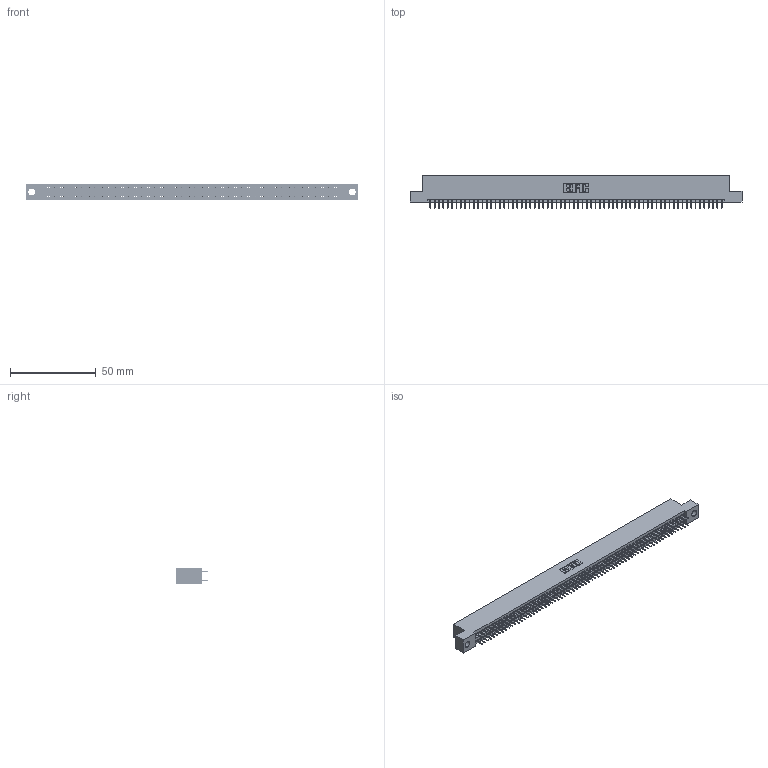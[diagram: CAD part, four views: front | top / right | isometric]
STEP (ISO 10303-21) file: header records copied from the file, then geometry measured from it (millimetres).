
FILE_DESCRIPTION (( 'STEP AP203' ), '1' );
FILE_NAME ('395-136-525-204.STEP', '2020-09-26T03:54:42', ( '' ), ( '' ), 'SwSTEP 2.0', 'SolidWorks 2020', '' );
FILE_SCHEMA (( 'CONFIG_CONTROL_DESIGN' ));
Length unit declared in the file: inch
Products named in the file (3): 345-292-001_345-293-125; 395-136-525-204; 345 Part_Flush Mounting Lugs - 0.156 Dia-TH
Assembly tree (137 placements, depth 2):
  395-136-525-204
    345 Part_Flush Mounting Lugs - 0.156 Dia-TH
    345-292-001_345-293-125  x136
Bounding box: 193.93 x 18.72 x 9.4 mm (x, y, z)
Volume: 18768.1 mm3; surface area: 27386.6 mm2
Topology: 137 solids, 137 shells, 7470 faces, 21149 edges, 13554 vertices
Faces by surface type: plane 5384, cylinder 2086
Entity records: 49931 total; most frequent: CARTESIAN_POINT 8344, ORIENTED_EDGE 8278, DIRECTION 7327, EDGE_CURVE 4139, LINE 3739, VECTOR 3739, VERTEX_POINT 2754, AXIS2_PLACEMENT_3D 1794
